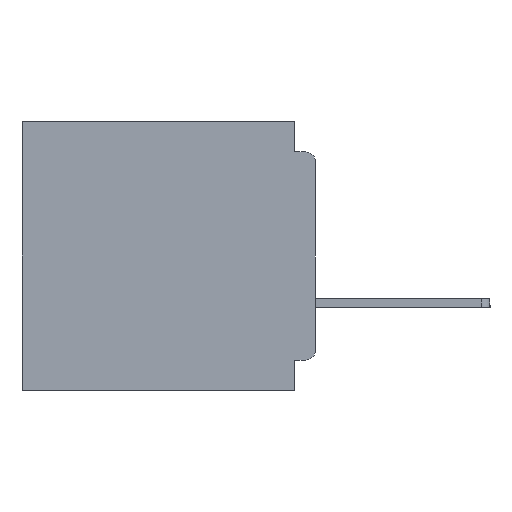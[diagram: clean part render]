
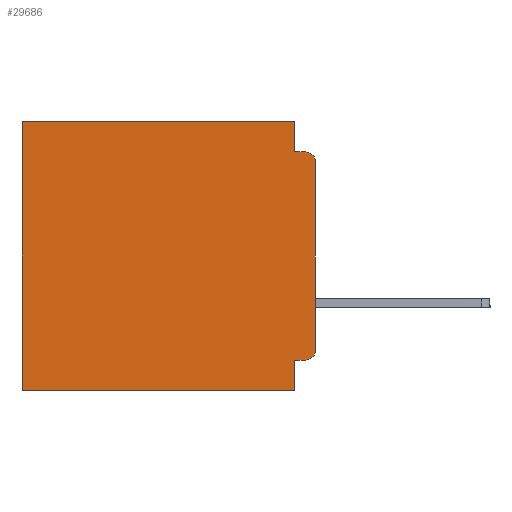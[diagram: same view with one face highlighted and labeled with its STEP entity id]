
A CAD part, left-side view. The second image highlights one B-rep face of the part: STEP entity #29686.
In plain terms, the highlighted planar face has unit normal (-1, 0, 0).
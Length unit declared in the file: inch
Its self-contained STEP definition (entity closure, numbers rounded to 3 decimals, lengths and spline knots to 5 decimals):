
#400 = VERTEX_POINT ( 'NONE', #6872 ) ;
#442 = ORIENTED_EDGE ( 'NONE', *, *, #22573, .F. ) ;
#593 = CARTESIAN_POINT ( 'NONE',  ( 0.3, 0.015, -0.34 ) ) ;
#603 = CARTESIAN_POINT ( 'NONE',  ( 0.3, 0.031, -0.4 ) ) ;
#786 = LINE ( 'NONE', #34936, #29458 ) ;
#971 = ORIENTED_EDGE ( 'NONE', *, *, #20048, .F. ) ;
#1001 = VERTEX_POINT ( 'NONE', #24609 ) ;
#1679 = CARTESIAN_POINT ( 'NONE',  ( 0.3, 0., -0.34 ) ) ;
#2258 = DIRECTION ( 'NONE',  ( 1., 0., 0. ) ) ;
#2263 = CARTESIAN_POINT ( 'NONE',  ( 0.3, 0., -0.045 ) ) ;
#2271 = ORIENTED_EDGE ( 'NONE', *, *, #2334, .T. ) ;
#2334 = EDGE_CURVE ( 'NONE', #45064, #9035, #786, .T. ) ;
#2596 = VERTEX_POINT ( 'NONE', #6089 ) ;
#4110 = VERTEX_POINT ( 'NONE', #30293 ) ;
#4394 = DIRECTION ( 'NONE',  ( 0., 0., -1. ) ) ;
#4400 = DIRECTION ( 'NONE',  ( 0., 0., -1. ) ) ;
#4477 = CARTESIAN_POINT ( 'NONE',  ( 0.3, 0.437, 0. ) ) ;
#5171 = ORIENTED_EDGE ( 'NONE', *, *, #7971, .F. ) ;
#5775 = VERTEX_POINT ( 'NONE', #39764 ) ;
#6060 = CARTESIAN_POINT ( 'NONE',  ( 0.3, 0.015, -0.355 ) ) ;
#6089 = CARTESIAN_POINT ( 'NONE',  ( 0.3, 0., -0.06 ) ) ;
#6667 = EDGE_CURVE ( 'NONE', #28384, #400, #20267, .T. ) ;
#6805 = CARTESIAN_POINT ( 'NONE',  ( 0.3, 0., -0.4 ) ) ;
#6872 = CARTESIAN_POINT ( 'NONE',  ( 0.3, 0.437, -0.4 ) ) ;
#7029 = EDGE_CURVE ( 'NONE', #2596, #15479, #34773, .T. ) ;
#7939 = DIRECTION ( 'NONE',  ( -1., 0., 0. ) ) ;
#7971 = EDGE_CURVE ( 'NONE', #7993, #4110, #11411, .T. ) ;
#7993 = VERTEX_POINT ( 'NONE', #6060 ) ;
#8535 = CARTESIAN_POINT ( 'NONE',  ( 0.3, 0., -0.4 ) ) ;
#8704 = CARTESIAN_POINT ( 'NONE',  ( 0.3, 0.437, -0.4 ) ) ;
#9035 = VERTEX_POINT ( 'NONE', #4477 ) ;
#10261 = VECTOR ( 'NONE', #28248, 39.37008 ) ;
#11411 = LINE ( 'NONE', #31982, #10261 ) ;
#11558 = ORIENTED_EDGE ( 'NONE', *, *, #27973, .F. ) ;
#12836 = AXIS2_PLACEMENT_3D ( 'NONE', #31957, #2258, #28381 ) ;
#13440 = DIRECTION ( 'NONE',  ( 0., 0., -1. ) ) ;
#15479 = VERTEX_POINT ( 'NONE', #1679 ) ;
#17020 = LINE ( 'NONE', #8704, #44239 ) ;
#17444 = CIRCLE ( 'NONE', #27070, 0.015 ) ;
#17563 = ORIENTED_EDGE ( 'NONE', *, *, #6667, .F. ) ;
#18365 = CARTESIAN_POINT ( 'NONE',  ( 0.3, 0.031, 0. ) ) ;
#19540 = EDGE_LOOP ( 'NONE', ( #39290, #24305, #11558, #442, #2271, #46998, #17563, #971, #5171, #27127 ) ) ;
#20048 = EDGE_CURVE ( 'NONE', #4110, #28384, #29925, .T. ) ;
#20267 = LINE ( 'NONE', #8535, #38870 ) ;
#22573 = EDGE_CURVE ( 'NONE', #45064, #5775, #34473, .T. ) ;
#24305 = ORIENTED_EDGE ( 'NONE', *, *, #41215, .T. ) ;
#24609 = CARTESIAN_POINT ( 'NONE',  ( 0.3, 0.015, -0.045 ) ) ;
#25383 = DIRECTION ( 'NONE',  ( 0., 0., -1. ) ) ;
#26744 = DIRECTION ( 'NONE',  ( -1., 0., 0. ) ) ;
#27070 = AXIS2_PLACEMENT_3D ( 'NONE', #593, #26744, #4394 ) ;
#27127 = ORIENTED_EDGE ( 'NONE', *, *, #36282, .T. ) ;
#27371 = DIRECTION ( 'NONE',  ( 0., 1., 0. ) ) ;
#27973 = EDGE_CURVE ( 'NONE', #5775, #1001, #29522, .T. ) ;
#28248 = DIRECTION ( 'NONE',  ( 0., 1., 0. ) ) ;
#28381 = DIRECTION ( 'NONE',  ( 0., 0., -1. ) ) ;
#28384 = VERTEX_POINT ( 'NONE', #45695 ) ;
#29458 = VECTOR ( 'NONE', #29965, 39.37008 ) ;
#29522 = LINE ( 'NONE', #2263, #30694 ) ;
#29686 = ADVANCED_FACE ( 'NONE', ( #46579 ), #43029, .F. ) ;
#29925 = LINE ( 'NONE', #603, #38568 ) ;
#29965 = DIRECTION ( 'NONE',  ( 0., 1., 0. ) ) ;
#30248 = CARTESIAN_POINT ( 'NONE',  ( 0.3, 0.015, -0.06 ) ) ;
#30293 = CARTESIAN_POINT ( 'NONE',  ( 0.3, 0.031, -0.355 ) ) ;
#30346 = AXIS2_PLACEMENT_3D ( 'NONE', #30248, #7939, #33930 ) ;
#30694 = VECTOR ( 'NONE', #32122, 39.37008 ) ;
#30782 = EDGE_CURVE ( 'NONE', #9035, #400, #17020, .T. ) ;
#31957 = CARTESIAN_POINT ( 'NONE',  ( 0.3, 0., -0.4 ) ) ;
#31982 = CARTESIAN_POINT ( 'NONE',  ( 0.3, 0., -0.355 ) ) ;
#32122 = DIRECTION ( 'NONE',  ( 0., -1., 0. ) ) ;
#32184 = CARTESIAN_POINT ( 'NONE',  ( 0.3, 0.031, 0. ) ) ;
#33357 = VECTOR ( 'NONE', #13440, 39.37008 ) ;
#33636 = VECTOR ( 'NONE', #25383, 39.37008 ) ;
#33930 = DIRECTION ( 'NONE',  ( 0., 0., -1. ) ) ;
#34473 = LINE ( 'NONE', #32184, #33357 ) ;
#34773 = LINE ( 'NONE', #6805, #33636 ) ;
#34936 = CARTESIAN_POINT ( 'NONE',  ( 0.3, 0., 0. ) ) ;
#36282 = EDGE_CURVE ( 'NONE', #7993, #15479, #17444, .T. ) ;
#38568 = VECTOR ( 'NONE', #4400, 39.37008 ) ;
#38870 = VECTOR ( 'NONE', #27371, 39.37008 ) ;
#39290 = ORIENTED_EDGE ( 'NONE', *, *, #7029, .F. ) ;
#39764 = CARTESIAN_POINT ( 'NONE',  ( 0.3, 0.031, -0.045 ) ) ;
#41215 = EDGE_CURVE ( 'NONE', #2596, #1001, #41261, .T. ) ;
#41261 = CIRCLE ( 'NONE', #30346, 0.015 ) ;
#42106 = DIRECTION ( 'NONE',  ( 0., 0., -1. ) ) ;
#43029 = PLANE ( 'NONE',  #12836 ) ;
#44239 = VECTOR ( 'NONE', #42106, 39.37008 ) ;
#45064 = VERTEX_POINT ( 'NONE', #18365 ) ;
#45695 = CARTESIAN_POINT ( 'NONE',  ( 0.3, 0.031, -0.4 ) ) ;
#46579 = FACE_OUTER_BOUND ( 'NONE', #19540, .T. ) ;
#46998 = ORIENTED_EDGE ( 'NONE', *, *, #30782, .T. ) ;
